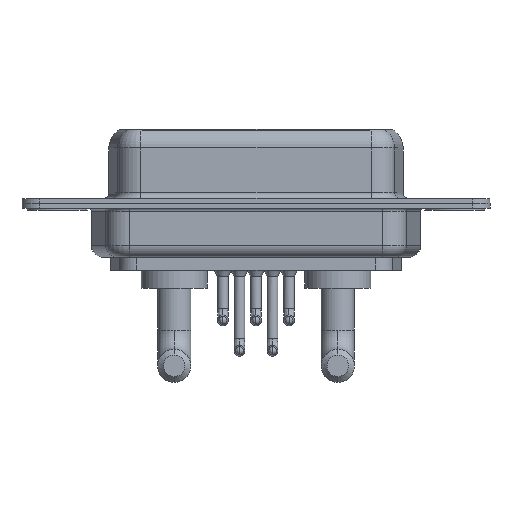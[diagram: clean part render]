
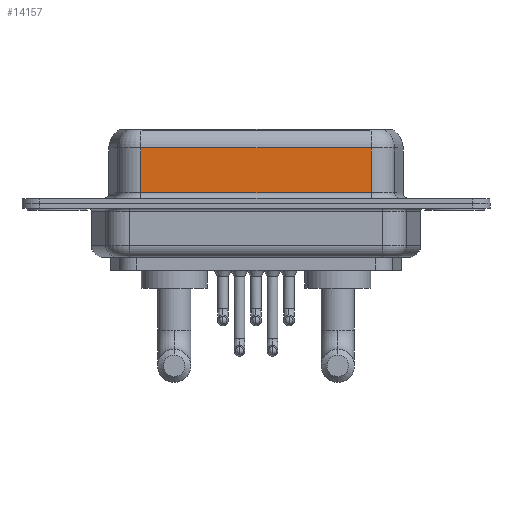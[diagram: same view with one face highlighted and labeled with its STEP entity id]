
A CAD part, front view. The second image highlights one B-rep face of the part: STEP entity #14157.
In plain terms, the highlighted planar face has unit normal (0, -1, 0).
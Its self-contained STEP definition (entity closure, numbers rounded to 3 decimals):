
#297 = ORIENTED_EDGE ( 'NONE', *, *, #1546, .F. ) ;
#444 = CARTESIAN_POINT ( 'NONE',  ( 26.287, -3.95, 6.4 ) ) ;
#986 = CARTESIAN_POINT ( 'NONE',  ( 7.013, -3.95, 6.4 ) ) ;
#1546 = EDGE_CURVE ( 'NONE', #7419, #3289, #6508, .T. ) ;
#2050 = EDGE_CURVE ( 'NONE', #5443, #12226, #11519, .T. ) ;
#2214 = DIRECTION ( 'NONE',  ( 0., 0., -1. ) ) ;
#2355 = FACE_OUTER_BOUND ( 'NONE', #5999, .T. ) ;
#3289 = VERTEX_POINT ( 'NONE', #12381 ) ;
#3321 = DIRECTION ( 'NONE',  ( 0., 0., -1. ) ) ;
#3922 = VECTOR ( 'NONE', #2214, 1000. ) ;
#4379 = CARTESIAN_POINT ( 'NONE',  ( 7.013, -3.95, 4.65 ) ) ;
#4546 = ORIENTED_EDGE ( 'NONE', *, *, #11957, .T. ) ;
#4802 = CARTESIAN_POINT ( 'NONE',  ( 26.287, -3.95, 0.9 ) ) ;
#5089 = PLANE ( 'NONE',  #6344 ) ;
#5348 = CARTESIAN_POINT ( 'NONE',  ( 26.287, -3.95, 4.65 ) ) ;
#5443 = VERTEX_POINT ( 'NONE', #4379 ) ;
#5999 = EDGE_LOOP ( 'NONE', ( #297, #4546, #7852, #8110 ) ) ;
#6234 = DIRECTION ( 'NONE',  ( 0., 1., 0. ) ) ;
#6344 = AXIS2_PLACEMENT_3D ( 'NONE', #444, #6234, #7465 ) ;
#6504 = LINE ( 'NONE', #10968, #8976 ) ;
#6508 = LINE ( 'NONE', #13694, #14933 ) ;
#7419 = VERTEX_POINT ( 'NONE', #5348 ) ;
#7465 = DIRECTION ( 'NONE',  ( 0., 0., 1. ) ) ;
#7852 = ORIENTED_EDGE ( 'NONE', *, *, #2050, .T. ) ;
#8110 = ORIENTED_EDGE ( 'NONE', *, *, #12591, .T. ) ;
#8976 = VECTOR ( 'NONE', #14543, 1000. ) ;
#9417 = CARTESIAN_POINT ( 'NONE',  ( 7.013, -3.95, 0.9 ) ) ;
#10968 = CARTESIAN_POINT ( 'NONE',  ( 26.287, -3.95, 4.65 ) ) ;
#11519 = LINE ( 'NONE', #986, #3922 ) ;
#11957 = EDGE_CURVE ( 'NONE', #7419, #5443, #6504, .T. ) ;
#12226 = VERTEX_POINT ( 'NONE', #9417 ) ;
#12381 = CARTESIAN_POINT ( 'NONE',  ( 26.287, -3.95, 0.9 ) ) ;
#12591 = EDGE_CURVE ( 'NONE', #12226, #3289, #15107, .T. ) ;
#12679 = VECTOR ( 'NONE', #12996, 1000. ) ;
#12996 = DIRECTION ( 'NONE',  ( 1., 0., 0. ) ) ;
#13694 = CARTESIAN_POINT ( 'NONE',  ( 26.287, -3.95, 6.4 ) ) ;
#14157 = ADVANCED_FACE ( 'NONE', ( #2355 ), #5089, .F. ) ;
#14543 = DIRECTION ( 'NONE',  ( -1., 0., 0. ) ) ;
#14933 = VECTOR ( 'NONE', #3321, 1000. ) ;
#15107 = LINE ( 'NONE', #4802, #12679 ) ;
